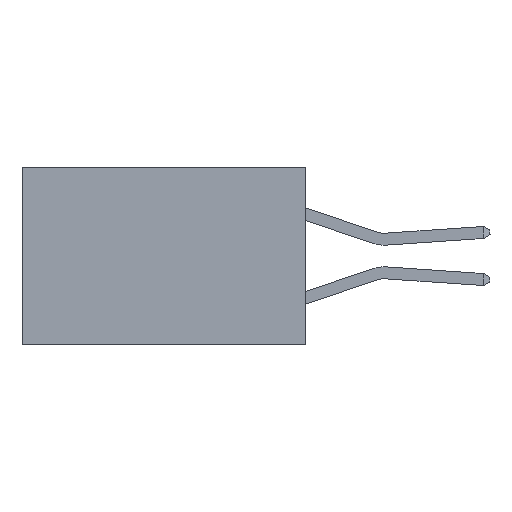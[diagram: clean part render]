
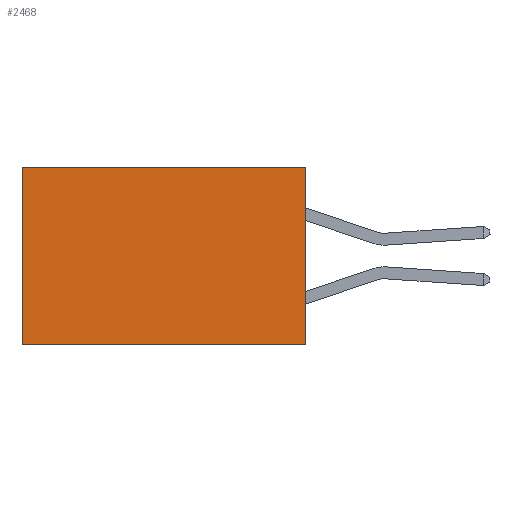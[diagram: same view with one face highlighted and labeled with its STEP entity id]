
A CAD part, left-side view. The second image highlights one B-rep face of the part: STEP entity #2468.
In plain terms, the highlighted planar face has unit normal (-1, 0, 0).
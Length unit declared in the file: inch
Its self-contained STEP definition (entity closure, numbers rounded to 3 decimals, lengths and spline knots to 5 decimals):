
#54 = VERTEX_POINT ( 'NONE', #8851 ) ;
#826 = CARTESIAN_POINT ( 'NONE',  ( 0.277, 0., 0. ) ) ;
#1478 = LINE ( 'NONE', #4337, #5795 ) ;
#1818 = VERTEX_POINT ( 'NONE', #11102 ) ;
#1966 = VECTOR ( 'NONE', #4945, 39.37008 ) ;
#2345 = ORIENTED_EDGE ( 'NONE', *, *, #10182, .T. ) ;
#2468 = ADVANCED_FACE ( 'NONE', ( #10189 ), #3693, .F. ) ;
#2516 = CARTESIAN_POINT ( 'NONE',  ( 0.277, 0., -0.37 ) ) ;
#2692 = DIRECTION ( 'NONE',  ( 0., 0., -1. ) ) ;
#2702 = DIRECTION ( 'NONE',  ( 1., 0., 0. ) ) ;
#3376 = ORIENTED_EDGE ( 'NONE', *, *, #4019, .T. ) ;
#3682 = EDGE_CURVE ( 'NONE', #11132, #54, #12449, .T. ) ;
#3693 = PLANE ( 'NONE',  #7269 ) ;
#4019 = EDGE_CURVE ( 'NONE', #4360, #1818, #1478, .T. ) ;
#4337 = CARTESIAN_POINT ( 'NONE',  ( 0.277, 0.59, -0.37 ) ) ;
#4360 = VERTEX_POINT ( 'NONE', #7459 ) ;
#4598 = VECTOR ( 'NONE', #7728, 39.37008 ) ;
#4945 = DIRECTION ( 'NONE',  ( 0., 0., -1. ) ) ;
#5413 = ORIENTED_EDGE ( 'NONE', *, *, #12213, .F. ) ;
#5795 = VECTOR ( 'NONE', #12135, 39.37008 ) ;
#6337 = ORIENTED_EDGE ( 'NONE', *, *, #3682, .F. ) ;
#6592 = LINE ( 'NONE', #10817, #11576 ) ;
#7269 = AXIS2_PLACEMENT_3D ( 'NONE', #2516, #2702, #2692 ) ;
#7459 = CARTESIAN_POINT ( 'NONE',  ( 0.277, 0.59, 0. ) ) ;
#7683 = CARTESIAN_POINT ( 'NONE',  ( 0.277, 0., -0.37 ) ) ;
#7728 = DIRECTION ( 'NONE',  ( 0., 1., 0. ) ) ;
#8102 = EDGE_LOOP ( 'NONE', ( #3376, #5413, #6337, #2345 ) ) ;
#8851 = CARTESIAN_POINT ( 'NONE',  ( 0.277, 0., -0.37 ) ) ;
#9182 = CARTESIAN_POINT ( 'NONE',  ( 0.277, 0., 0. ) ) ;
#10182 = EDGE_CURVE ( 'NONE', #11132, #4360, #12215, .T. ) ;
#10189 = FACE_OUTER_BOUND ( 'NONE', #8102, .T. ) ;
#10817 = CARTESIAN_POINT ( 'NONE',  ( 0.277, 0., -0.37 ) ) ;
#11102 = CARTESIAN_POINT ( 'NONE',  ( 0.277, 0.59, -0.37 ) ) ;
#11132 = VERTEX_POINT ( 'NONE', #9182 ) ;
#11576 = VECTOR ( 'NONE', #11776, 39.37008 ) ;
#11776 = DIRECTION ( 'NONE',  ( 0., 1., 0. ) ) ;
#12135 = DIRECTION ( 'NONE',  ( 0., 0., -1. ) ) ;
#12213 = EDGE_CURVE ( 'NONE', #54, #1818, #6592, .T. ) ;
#12215 = LINE ( 'NONE', #826, #4598 ) ;
#12449 = LINE ( 'NONE', #7683, #1966 ) ;
